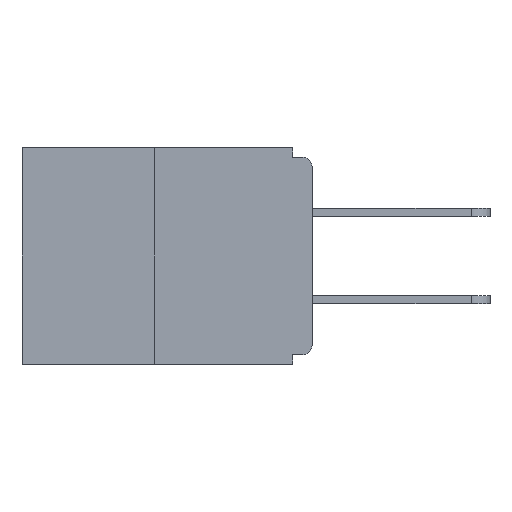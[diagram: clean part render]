
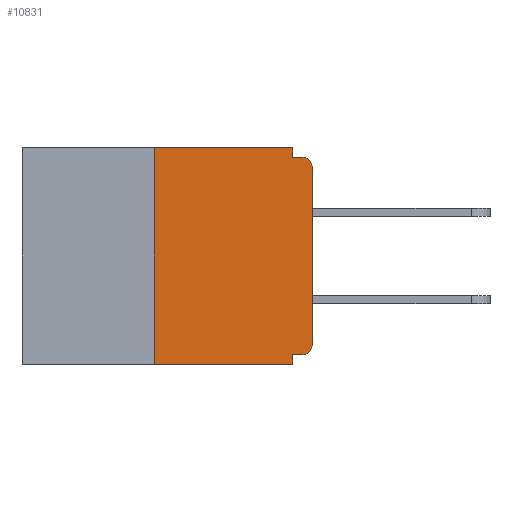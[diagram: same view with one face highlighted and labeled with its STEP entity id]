
A CAD part, left-side view. The second image highlights one B-rep face of the part: STEP entity #10831.
In plain terms, the highlighted planar face has unit normal (-1, 0, 0).
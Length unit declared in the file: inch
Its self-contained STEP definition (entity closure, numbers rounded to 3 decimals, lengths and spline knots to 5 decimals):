
#32 = CARTESIAN_POINT ( 'NONE',  ( 0., 0.031, -0.015 ) ) ;
#79 = EDGE_LOOP ( 'NONE', ( #10123, #15378, #3491, #12182, #8316, #5880, #1235, #9898, #15804, #15459 ) ) ;
#102 = FACE_OUTER_BOUND ( 'NONE', #79, .T. ) ;
#154 = CARTESIAN_POINT ( 'NONE',  ( 0., 0., -0.015 ) ) ;
#348 = CARTESIAN_POINT ( 'NONE',  ( 0., 0., -0.03 ) ) ;
#537 = VECTOR ( 'NONE', #10268, 39.37008 ) ;
#648 = VECTOR ( 'NONE', #15437, 39.37008 ) ;
#707 = LINE ( 'NONE', #11184, #5992 ) ;
#756 = DIRECTION ( 'NONE',  ( 0., 0., -1. ) ) ;
#798 = CARTESIAN_POINT ( 'NONE',  ( 0., 0.015, -0.03 ) ) ;
#1235 = ORIENTED_EDGE ( 'NONE', *, *, #11015, .T. ) ;
#1340 = CARTESIAN_POINT ( 'NONE',  ( 0., 0.46, -0.343 ) ) ;
#1431 = CARTESIAN_POINT ( 'NONE',  ( 0., 0.25, -0.343 ) ) ;
#1441 = EDGE_CURVE ( 'NONE', #2679, #11396, #4525, .T. ) ;
#2287 = DIRECTION ( 'NONE',  ( -1., 0., 0. ) ) ;
#2651 = VECTOR ( 'NONE', #4085, 39.37008 ) ;
#2679 = VERTEX_POINT ( 'NONE', #10379 ) ;
#3491 = ORIENTED_EDGE ( 'NONE', *, *, #12459, .T. ) ;
#3509 = EDGE_CURVE ( 'NONE', #10086, #7583, #11722, .T. ) ;
#3518 = DIRECTION ( 'NONE',  ( 0., 0., 1. ) ) ;
#3867 = DIRECTION ( 'NONE',  ( 0., 0., -1. ) ) ;
#4085 = DIRECTION ( 'NONE',  ( 0., 1., 0. ) ) ;
#4163 = DIRECTION ( 'NONE',  ( 0., 0., -1. ) ) ;
#4346 = CARTESIAN_POINT ( 'NONE',  ( 0., 0.031, -0.343 ) ) ;
#4407 = VERTEX_POINT ( 'NONE', #8513 ) ;
#4525 = LINE ( 'NONE', #16662, #9188 ) ;
#4759 = VERTEX_POINT ( 'NONE', #1431 ) ;
#4846 = AXIS2_PLACEMENT_3D ( 'NONE', #14349, #10514, #4163 ) ;
#5174 = VERTEX_POINT ( 'NONE', #32 ) ;
#5256 = PLANE ( 'NONE',  #4846 ) ;
#5481 = AXIS2_PLACEMENT_3D ( 'NONE', #798, #12481, #756 ) ;
#5880 = ORIENTED_EDGE ( 'NONE', *, *, #10433, .T. ) ;
#5992 = VECTOR ( 'NONE', #3518, 39.37008 ) ;
#6018 = VERTEX_POINT ( 'NONE', #16144 ) ;
#6042 = CARTESIAN_POINT ( 'NONE',  ( 0., 0.031, 0. ) ) ;
#6223 = DIRECTION ( 'NONE',  ( 0., 0., -1. ) ) ;
#6311 = CARTESIAN_POINT ( 'NONE',  ( 0., 0.031, 0. ) ) ;
#6421 = CARTESIAN_POINT ( 'NONE',  ( 0., 0., -0.328 ) ) ;
#6546 = LINE ( 'NONE', #1340, #648 ) ;
#7084 = VECTOR ( 'NONE', #12378, 39.37008 ) ;
#7336 = CIRCLE ( 'NONE', #5481, 0.015 ) ;
#7345 = CARTESIAN_POINT ( 'NONE',  ( 0., 0., -0.313 ) ) ;
#7527 = EDGE_CURVE ( 'NONE', #16509, #4407, #7336, .T. ) ;
#7583 = VERTEX_POINT ( 'NONE', #6042 ) ;
#7952 = VECTOR ( 'NONE', #16269, 39.37008 ) ;
#8231 = CIRCLE ( 'NONE', #11966, 0.015 ) ;
#8316 = ORIENTED_EDGE ( 'NONE', *, *, #13539, .F. ) ;
#8513 = CARTESIAN_POINT ( 'NONE',  ( 0., 0.015, -0.015 ) ) ;
#8532 = CARTESIAN_POINT ( 'NONE',  ( 0., 0.46, 0. ) ) ;
#9188 = VECTOR ( 'NONE', #3867, 39.37008 ) ;
#9898 = ORIENTED_EDGE ( 'NONE', *, *, #7527, .T. ) ;
#10086 = VERTEX_POINT ( 'NONE', #13312 ) ;
#10123 = ORIENTED_EDGE ( 'NONE', *, *, #3509, .F. ) ;
#10268 = DIRECTION ( 'NONE',  ( 0., -1., 0. ) ) ;
#10272 = EDGE_CURVE ( 'NONE', #5174, #4407, #12846, .T. ) ;
#10379 = CARTESIAN_POINT ( 'NONE',  ( 0., 0.031, -0.328 ) ) ;
#10433 = EDGE_CURVE ( 'NONE', #6018, #15420, #8231, .T. ) ;
#10514 = DIRECTION ( 'NONE',  ( 1., 0., 0. ) ) ;
#10831 = ADVANCED_FACE ( 'NONE', ( #102 ), #5256, .F. ) ;
#10985 = EDGE_CURVE ( 'NONE', #7583, #5174, #14015, .T. ) ;
#11015 = EDGE_CURVE ( 'NONE', #15420, #16509, #707, .T. ) ;
#11184 = CARTESIAN_POINT ( 'NONE',  ( 0., 0., 0. ) ) ;
#11302 = DIRECTION ( 'NONE',  ( 0., 0., -1. ) ) ;
#11396 = VERTEX_POINT ( 'NONE', #4346 ) ;
#11442 = CARTESIAN_POINT ( 'NONE',  ( 0., 0.015, -0.313 ) ) ;
#11722 = LINE ( 'NONE', #8532, #7084 ) ;
#11787 = LINE ( 'NONE', #16151, #7952 ) ;
#11966 = AXIS2_PLACEMENT_3D ( 'NONE', #11442, #2287, #6223 ) ;
#12098 = EDGE_CURVE ( 'NONE', #4759, #10086, #11787, .T. ) ;
#12182 = ORIENTED_EDGE ( 'NONE', *, *, #1441, .F. ) ;
#12378 = DIRECTION ( 'NONE',  ( 0., -1., 0. ) ) ;
#12459 = EDGE_CURVE ( 'NONE', #4759, #11396, #6546, .T. ) ;
#12481 = DIRECTION ( 'NONE',  ( -1., 0., 0. ) ) ;
#12516 = LINE ( 'NONE', #6421, #2651 ) ;
#12846 = LINE ( 'NONE', #154, #537 ) ;
#13312 = CARTESIAN_POINT ( 'NONE',  ( 0., 0.25, 0. ) ) ;
#13539 = EDGE_CURVE ( 'NONE', #6018, #2679, #12516, .T. ) ;
#13618 = VECTOR ( 'NONE', #11302, 39.37008 ) ;
#14015 = LINE ( 'NONE', #6311, #13618 ) ;
#14349 = CARTESIAN_POINT ( 'NONE',  ( 0., 0.46, 0. ) ) ;
#15378 = ORIENTED_EDGE ( 'NONE', *, *, #12098, .F. ) ;
#15420 = VERTEX_POINT ( 'NONE', #7345 ) ;
#15437 = DIRECTION ( 'NONE',  ( 0., -1., 0. ) ) ;
#15459 = ORIENTED_EDGE ( 'NONE', *, *, #10985, .F. ) ;
#15804 = ORIENTED_EDGE ( 'NONE', *, *, #10272, .F. ) ;
#16144 = CARTESIAN_POINT ( 'NONE',  ( 0., 0.015, -0.328 ) ) ;
#16151 = CARTESIAN_POINT ( 'NONE',  ( 0., 0.25, 0. ) ) ;
#16269 = DIRECTION ( 'NONE',  ( 0., 0., 1. ) ) ;
#16509 = VERTEX_POINT ( 'NONE', #348 ) ;
#16662 = CARTESIAN_POINT ( 'NONE',  ( 0., 0.031, -0.343 ) ) ;
